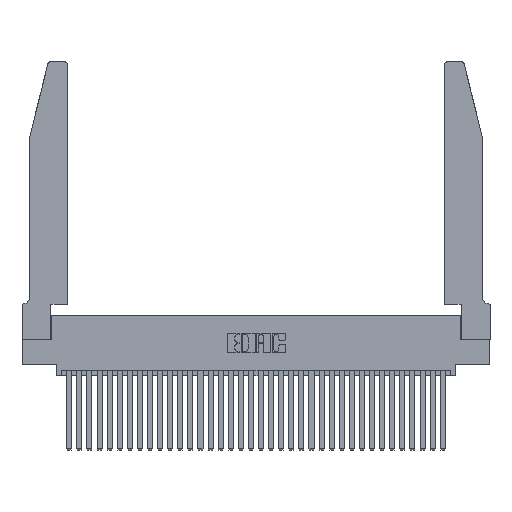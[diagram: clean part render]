
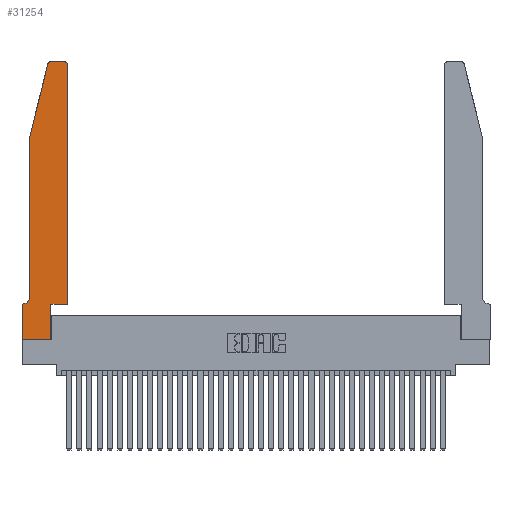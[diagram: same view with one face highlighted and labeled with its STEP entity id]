
A CAD part, top view. The second image highlights one B-rep face of the part: STEP entity #31254.
In plain terms, the highlighted planar face has unit normal (0, 0, 1).
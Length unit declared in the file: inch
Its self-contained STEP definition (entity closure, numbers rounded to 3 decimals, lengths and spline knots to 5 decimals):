
#328 = CARTESIAN_POINT ( 'NONE',  ( 0.0055, 0.35, 0.37 ) ) ;
#547 = CARTESIAN_POINT ( 'NONE',  ( 0.0755, 2., 0.37 ) ) ;
#619 = EDGE_CURVE ( 'NONE', #30515, #26688, #34004, .T. ) ;
#649 = ORIENTED_EDGE ( 'NONE', *, *, #2642, .T. ) ;
#992 = CARTESIAN_POINT ( 'NONE',  ( 0.0755, 2., 0.37 ) ) ;
#1004 = VECTOR ( 'NONE', #32753, 39.37008 ) ;
#1766 = LINE ( 'NONE', #29220, #5990 ) ;
#2585 = CARTESIAN_POINT ( 'NONE',  ( 0.0755, 0.42, 0.37 ) ) ;
#2642 = EDGE_CURVE ( 'NONE', #20767, #6458, #28544, .T. ) ;
#3339 = CARTESIAN_POINT ( 'NONE',  ( 0.4505, 0.35, 0.37 ) ) ;
#3353 = EDGE_CURVE ( 'NONE', #26691, #20767, #7352, .T. ) ;
#3839 = DIRECTION ( 'NONE',  ( 0., -1., 0. ) ) ;
#3922 = CARTESIAN_POINT ( 'NONE',  ( 0.2865, 0.35, 0.37 ) ) ;
#4955 = LINE ( 'NONE', #547, #32866 ) ;
#5028 = EDGE_CURVE ( 'NONE', #26688, #15135, #28396, .T. ) ;
#5170 = ORIENTED_EDGE ( 'NONE', *, *, #619, .T. ) ;
#5528 = VERTEX_POINT ( 'NONE', #5847 ) ;
#5847 = CARTESIAN_POINT ( 'NONE',  ( 0.0755, 2., 0.37 ) ) ;
#5873 = DIRECTION ( 'NONE',  ( 0., -1., 0. ) ) ;
#5990 = VECTOR ( 'NONE', #13183, 39.37008 ) ;
#6458 = VERTEX_POINT ( 'NONE', #8160 ) ;
#6531 = CARTESIAN_POINT ( 'NONE',  ( 0.0055, 0.42, 0.37 ) ) ;
#6632 = DIRECTION ( 'NONE',  ( 0., 1., 0. ) ) ;
#6693 = AXIS2_PLACEMENT_3D ( 'NONE', #34749, #28806, #10369 ) ;
#6792 = ORIENTED_EDGE ( 'NONE', *, *, #25947, .T. ) ;
#7115 = CARTESIAN_POINT ( 'NONE',  ( 0., 0., 0.37 ) ) ;
#7352 = CIRCLE ( 'NONE', #17346, 0.07 ) ;
#7939 = EDGE_LOOP ( 'NONE', ( #26515, #22625, #8357, #9115, #30996, #649, #11602, #14590, #6792, #26222, #5170, #22519 ) ) ;
#8160 = CARTESIAN_POINT ( 'NONE',  ( 0., 0.35, 0.37 ) ) ;
#8168 = DIRECTION ( 'NONE',  ( 0., 0., 1. ) ) ;
#8357 = ORIENTED_EDGE ( 'NONE', *, *, #20245, .T. ) ;
#8395 = VECTOR ( 'NONE', #3839, 39.37008 ) ;
#9115 = ORIENTED_EDGE ( 'NONE', *, *, #19151, .T. ) ;
#9235 = CARTESIAN_POINT ( 'NONE',  ( 0.2605, 2.75, 0.37 ) ) ;
#9340 = LINE ( 'NONE', #9235, #29243 ) ;
#9669 = VERTEX_POINT ( 'NONE', #7115 ) ;
#10155 = AXIS2_PLACEMENT_3D ( 'NONE', #20408, #25890, #31348 ) ;
#10369 = DIRECTION ( 'NONE',  ( 1., 0., 0. ) ) ;
#10913 = AXIS2_PLACEMENT_3D ( 'NONE', #11257, #8168, #30170 ) ;
#11127 = EDGE_CURVE ( 'NONE', #23803, #19160, #23546, .T. ) ;
#11257 = CARTESIAN_POINT ( 'NONE',  ( 0., 0.35, 0.37 ) ) ;
#11602 = ORIENTED_EDGE ( 'NONE', *, *, #24848, .T. ) ;
#11916 = DIRECTION ( 'NONE',  ( 0., 0., -1. ) ) ;
#12071 = CARTESIAN_POINT ( 'NONE',  ( 0.25487, 2.72718, 0.37 ) ) ;
#12479 = VECTOR ( 'NONE', #15387, 39.37008 ) ;
#13183 = DIRECTION ( 'NONE',  ( 1., 0., 0. ) ) ;
#13287 = LINE ( 'NONE', #21955, #33558 ) ;
#13973 = CARTESIAN_POINT ( 'NONE',  ( 0.0755, 0.35, 0.37 ) ) ;
#14365 = LINE ( 'NONE', #992, #8395 ) ;
#14590 = ORIENTED_EDGE ( 'NONE', *, *, #29332, .T. ) ;
#14857 = DIRECTION ( 'NONE',  ( -1., 0., 0. ) ) ;
#15135 = VERTEX_POINT ( 'NONE', #23919 ) ;
#15387 = DIRECTION ( 'NONE',  ( 0., 1., 0. ) ) ;
#17090 = DIRECTION ( 'NONE',  ( -1., 0., 0. ) ) ;
#17151 = VECTOR ( 'NONE', #6632, 39.37008 ) ;
#17346 = AXIS2_PLACEMENT_3D ( 'NONE', #6531, #11916, #14857 ) ;
#18773 = CARTESIAN_POINT ( 'NONE',  ( 0.4505, 2.72, 0.37 ) ) ;
#19151 = EDGE_CURVE ( 'NONE', #5528, #26691, #14365, .T. ) ;
#19160 = VERTEX_POINT ( 'NONE', #12071 ) ;
#19462 = DIRECTION ( 'NONE',  ( -0.239, -0.971, 0. ) ) ;
#19650 = LINE ( 'NONE', #3922, #17151 ) ;
#19772 = FACE_OUTER_BOUND ( 'NONE', #7939, .T. ) ;
#19843 = VERTEX_POINT ( 'NONE', #21525 ) ;
#20245 = EDGE_CURVE ( 'NONE', #19160, #5528, #4955, .T. ) ;
#20408 = CARTESIAN_POINT ( 'NONE',  ( 0.284, 2.72, 0.37 ) ) ;
#20767 = VERTEX_POINT ( 'NONE', #328 ) ;
#20770 = CARTESIAN_POINT ( 'NONE',  ( 0., 0., 0.37 ) ) ;
#21525 = CARTESIAN_POINT ( 'NONE',  ( 0.2865, 0., 0.37 ) ) ;
#21955 = CARTESIAN_POINT ( 'NONE',  ( 0.4505, 0.35, 0.37 ) ) ;
#22457 = CARTESIAN_POINT ( 'NONE',  ( 0.284, 2.75, 0.37 ) ) ;
#22519 = ORIENTED_EDGE ( 'NONE', *, *, #5028, .T. ) ;
#22625 = ORIENTED_EDGE ( 'NONE', *, *, #11127, .T. ) ;
#23546 = CIRCLE ( 'NONE', #10155, 0.03 ) ;
#23803 = VERTEX_POINT ( 'NONE', #22457 ) ;
#23919 = CARTESIAN_POINT ( 'NONE',  ( 0.4205, 2.75, 0.37 ) ) ;
#24828 = VERTEX_POINT ( 'NONE', #25773 ) ;
#24848 = EDGE_CURVE ( 'NONE', #6458, #9669, #30368, .T. ) ;
#25773 = CARTESIAN_POINT ( 'NONE',  ( 0.2865, 0.35, 0.37 ) ) ;
#25890 = DIRECTION ( 'NONE',  ( 0., 0., 1. ) ) ;
#25947 = EDGE_CURVE ( 'NONE', #19843, #24828, #19650, .T. ) ;
#26222 = ORIENTED_EDGE ( 'NONE', *, *, #34441, .T. ) ;
#26515 = ORIENTED_EDGE ( 'NONE', *, *, #29068, .T. ) ;
#26688 = VERTEX_POINT ( 'NONE', #18773 ) ;
#26691 = VERTEX_POINT ( 'NONE', #2585 ) ;
#27291 = DIRECTION ( 'NONE',  ( 1., 0., 0. ) ) ;
#27301 = PLANE ( 'NONE',  #10913 ) ;
#28396 = CIRCLE ( 'NONE', #6693, 0.03 ) ;
#28544 = LINE ( 'NONE', #13973, #1004 ) ;
#28806 = DIRECTION ( 'NONE',  ( 0., 0., 1. ) ) ;
#29068 = EDGE_CURVE ( 'NONE', #15135, #23803, #9340, .T. ) ;
#29220 = CARTESIAN_POINT ( 'NONE',  ( 0., 0., 0.37 ) ) ;
#29243 = VECTOR ( 'NONE', #17090, 39.37008 ) ;
#29332 = EDGE_CURVE ( 'NONE', #9669, #19843, #1766, .T. ) ;
#30170 = DIRECTION ( 'NONE',  ( 1., 0., 0. ) ) ;
#30368 = LINE ( 'NONE', #20770, #31626 ) ;
#30515 = VERTEX_POINT ( 'NONE', #3339 ) ;
#30996 = ORIENTED_EDGE ( 'NONE', *, *, #3353, .T. ) ;
#31254 = ADVANCED_FACE ( 'NONE', ( #19772 ), #27301, .T. ) ;
#31348 = DIRECTION ( 'NONE',  ( 1., 0., 0. ) ) ;
#31626 = VECTOR ( 'NONE', #5873, 39.37008 ) ;
#32753 = DIRECTION ( 'NONE',  ( -1., 0., 0. ) ) ;
#32866 = VECTOR ( 'NONE', #19462, 39.37008 ) ;
#33558 = VECTOR ( 'NONE', #27291, 39.37008 ) ;
#34004 = LINE ( 'NONE', #34654, #12479 ) ;
#34441 = EDGE_CURVE ( 'NONE', #24828, #30515, #13287, .T. ) ;
#34654 = CARTESIAN_POINT ( 'NONE',  ( 0.4505, 0.35, 0.37 ) ) ;
#34749 = CARTESIAN_POINT ( 'NONE',  ( 0.4205, 2.72, 0.37 ) ) ;
